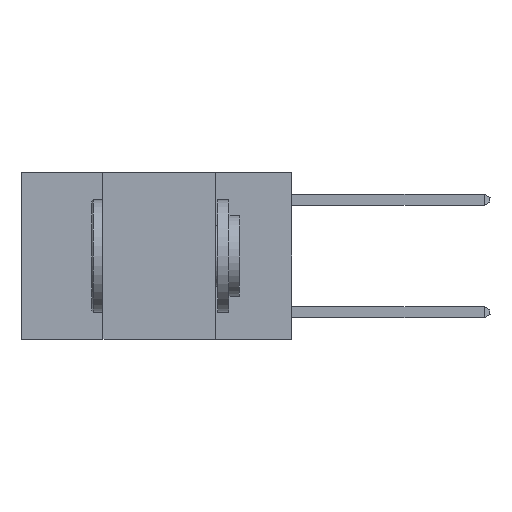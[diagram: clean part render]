
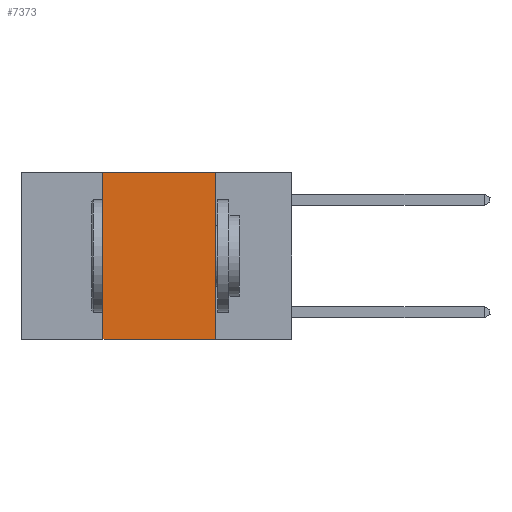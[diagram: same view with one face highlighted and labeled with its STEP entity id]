
A CAD part, left-side view. The second image highlights one B-rep face of the part: STEP entity #7373.
In plain terms, the highlighted planar face has unit normal (-1, 0, 0).
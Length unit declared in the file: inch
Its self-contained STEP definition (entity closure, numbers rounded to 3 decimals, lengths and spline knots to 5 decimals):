
#215 = VECTOR ( 'NONE', #7663, 39.37008 ) ;
#331 = EDGE_LOOP ( 'NONE', ( #11691, #8055, #2397, #13491 ) ) ;
#906 = FACE_OUTER_BOUND ( 'NONE', #331, .T. ) ;
#979 = CARTESIAN_POINT ( 'NONE',  ( 0., 0.17, -0.37 ) ) ;
#2015 = VECTOR ( 'NONE', #13128, 39.37008 ) ;
#2397 = ORIENTED_EDGE ( 'NONE', *, *, #4504, .F. ) ;
#2645 = LINE ( 'NONE', #4130, #215 ) ;
#3090 = AXIS2_PLACEMENT_3D ( 'NONE', #3296, #8136, #14695 ) ;
#3296 = CARTESIAN_POINT ( 'NONE',  ( 0., 0.6, 0. ) ) ;
#3396 = EDGE_CURVE ( 'NONE', #7702, #4969, #15991, .T. ) ;
#4130 = CARTESIAN_POINT ( 'NONE',  ( 0., 0.6, 0. ) ) ;
#4504 = EDGE_CURVE ( 'NONE', #9260, #15267, #9156, .T. ) ;
#4764 = CARTESIAN_POINT ( 'NONE',  ( 0., 0.17, 0. ) ) ;
#4969 = VERTEX_POINT ( 'NONE', #979 ) ;
#5499 = CARTESIAN_POINT ( 'NONE',  ( 0., 0.42, -0.37 ) ) ;
#6201 = VECTOR ( 'NONE', #14656, 39.37008 ) ;
#7050 = PLANE ( 'NONE',  #3090 ) ;
#7373 = ADVANCED_FACE ( 'NONE', ( #906 ), #7050, .F. ) ;
#7663 = DIRECTION ( 'NONE',  ( 0., -1., 0. ) ) ;
#7702 = VERTEX_POINT ( 'NONE', #13862 ) ;
#7798 = CARTESIAN_POINT ( 'NONE',  ( 0., 0.42, 0. ) ) ;
#7965 = DIRECTION ( 'NONE',  ( 0., 0., 1. ) ) ;
#8055 = ORIENTED_EDGE ( 'NONE', *, *, #12366, .F. ) ;
#8136 = DIRECTION ( 'NONE',  ( 1., 0., 0. ) ) ;
#9156 = LINE ( 'NONE', #13058, #13016 ) ;
#9260 = VERTEX_POINT ( 'NONE', #5499 ) ;
#11521 = EDGE_CURVE ( 'NONE', #9260, #4969, #12121, .T. ) ;
#11691 = ORIENTED_EDGE ( 'NONE', *, *, #3396, .F. ) ;
#12121 = LINE ( 'NONE', #13497, #6201 ) ;
#12366 = EDGE_CURVE ( 'NONE', #15267, #7702, #2645, .T. ) ;
#13016 = VECTOR ( 'NONE', #7965, 39.37008 ) ;
#13058 = CARTESIAN_POINT ( 'NONE',  ( 0., 0.42, 0. ) ) ;
#13128 = DIRECTION ( 'NONE',  ( 0., 0., -1. ) ) ;
#13491 = ORIENTED_EDGE ( 'NONE', *, *, #11521, .T. ) ;
#13497 = CARTESIAN_POINT ( 'NONE',  ( 0., 0.6, -0.37 ) ) ;
#13862 = CARTESIAN_POINT ( 'NONE',  ( 0., 0.17, 0. ) ) ;
#14656 = DIRECTION ( 'NONE',  ( 0., -1., 0. ) ) ;
#14695 = DIRECTION ( 'NONE',  ( 0., 0., -1. ) ) ;
#15267 = VERTEX_POINT ( 'NONE', #7798 ) ;
#15991 = LINE ( 'NONE', #4764, #2015 ) ;
